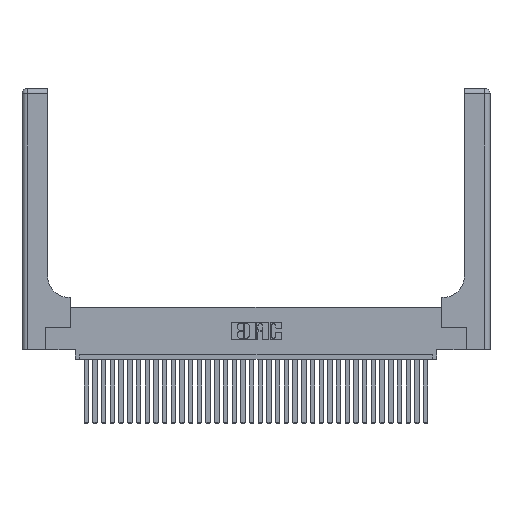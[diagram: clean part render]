
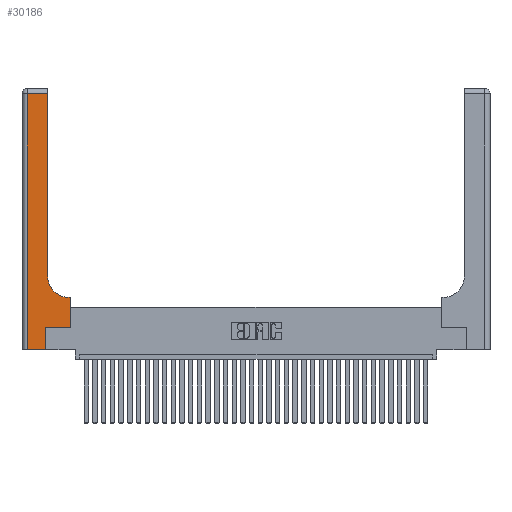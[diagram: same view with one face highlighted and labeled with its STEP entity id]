
A CAD part, top view. The second image highlights one B-rep face of the part: STEP entity #30186.
In plain terms, the highlighted planar face has unit normal (0, 0, 1).
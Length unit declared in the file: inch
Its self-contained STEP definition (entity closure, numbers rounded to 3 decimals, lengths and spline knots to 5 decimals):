
#1551 = PLANE ( 'NONE',  #24170 ) ;
#1641 = FACE_OUTER_BOUND ( 'NONE', #23028, .T. ) ;
#1851 = CIRCLE ( 'NONE', #33750, 0.25 ) ;
#2514 = ORIENTED_EDGE ( 'NONE', *, *, #33948, .T. ) ;
#2633 = EDGE_CURVE ( 'NONE', #8503, #35293, #25731, .T. ) ;
#3363 = CARTESIAN_POINT ( 'NONE',  ( 0.2915, 3., 0.37 ) ) ;
#3976 = ORIENTED_EDGE ( 'NONE', *, *, #13596, .T. ) ;
#4954 = EDGE_CURVE ( 'NONE', #15916, #24960, #19930, .T. ) ;
#4958 = EDGE_CURVE ( 'NONE', #7958, #14568, #5290, .T. ) ;
#4986 = DIRECTION ( 'NONE',  ( 0., 0., -1. ) ) ;
#5290 = LINE ( 'NONE', #32312, #18690 ) ;
#5787 = LINE ( 'NONE', #25757, #12323 ) ;
#6427 = LINE ( 'NONE', #31653, #23250 ) ;
#6730 = EDGE_CURVE ( 'NONE', #35293, #18492, #1851, .T. ) ;
#6784 = CARTESIAN_POINT ( 'NONE',  ( 0.06, 0., 0.37 ) ) ;
#6954 = CARTESIAN_POINT ( 'NONE',  ( 0.2915, 0.85, 0.37 ) ) ;
#7958 = VERTEX_POINT ( 'NONE', #24317 ) ;
#8503 = VERTEX_POINT ( 'NONE', #20651 ) ;
#8727 = DIRECTION ( 'NONE',  ( 0., 1., 0. ) ) ;
#9308 = ORIENTED_EDGE ( 'NONE', *, *, #25442, .T. ) ;
#9328 = CARTESIAN_POINT ( 'NONE',  ( 0.2915, 2.94, 0.37 ) ) ;
#9330 = ORIENTED_EDGE ( 'NONE', *, *, #6730, .T. ) ;
#9732 = CARTESIAN_POINT ( 'NONE',  ( 0.06, 2.94, 0.37 ) ) ;
#9828 = VECTOR ( 'NONE', #20749, 39.37008 ) ;
#9844 = CARTESIAN_POINT ( 'NONE',  ( 0., 3., 0.37 ) ) ;
#11902 = CARTESIAN_POINT ( 'NONE',  ( 0., 0., 0.37 ) ) ;
#12200 = ORIENTED_EDGE ( 'NONE', *, *, #29926, .T. ) ;
#12323 = VECTOR ( 'NONE', #31496, 39.37008 ) ;
#13596 = EDGE_CURVE ( 'NONE', #18492, #30036, #19755, .T. ) ;
#14226 = DIRECTION ( 'NONE',  ( -1., 0., 0. ) ) ;
#14568 = VERTEX_POINT ( 'NONE', #30795 ) ;
#15698 = CARTESIAN_POINT ( 'NONE',  ( 0.2915, 0.6, 0.37 ) ) ;
#15916 = VERTEX_POINT ( 'NONE', #9732 ) ;
#15969 = CARTESIAN_POINT ( 'NONE',  ( 0.5415, 0.6, 0.37 ) ) ;
#16258 = DIRECTION ( 'NONE',  ( 1., 0., 0. ) ) ;
#18492 = VERTEX_POINT ( 'NONE', #6954 ) ;
#18643 = CARTESIAN_POINT ( 'NONE',  ( 0.5585, 0.25, 0.37 ) ) ;
#18690 = VECTOR ( 'NONE', #21539, 39.37008 ) ;
#19100 = CARTESIAN_POINT ( 'NONE',  ( 0.5415, 0.85, 0.37 ) ) ;
#19532 = EDGE_CURVE ( 'NONE', #30036, #15916, #6427, .T. ) ;
#19755 = LINE ( 'NONE', #3363, #32232 ) ;
#19899 = VERTEX_POINT ( 'NONE', #35441 ) ;
#19930 = LINE ( 'NONE', #28637, #35369 ) ;
#20559 = LINE ( 'NONE', #11902, #32533 ) ;
#20651 = CARTESIAN_POINT ( 'NONE',  ( 0.5585, 0.6, 0.37 ) ) ;
#20749 = DIRECTION ( 'NONE',  ( -1., 0., 0. ) ) ;
#21539 = DIRECTION ( 'NONE',  ( 0., 1., 0. ) ) ;
#22475 = ORIENTED_EDGE ( 'NONE', *, *, #19532, .T. ) ;
#23028 = EDGE_LOOP ( 'NONE', ( #3976, #22475, #32896, #12200, #29825, #2514, #9308, #23126, #9330 ) ) ;
#23126 = ORIENTED_EDGE ( 'NONE', *, *, #2633, .T. ) ;
#23250 = VECTOR ( 'NONE', #23511, 39.37008 ) ;
#23511 = DIRECTION ( 'NONE',  ( -1., 0., 0. ) ) ;
#23925 = VECTOR ( 'NONE', #30034, 39.37008 ) ;
#24170 = AXIS2_PLACEMENT_3D ( 'NONE', #9844, #4986, #14226 ) ;
#24317 = CARTESIAN_POINT ( 'NONE',  ( 0.269, 0., 0.37 ) ) ;
#24960 = VERTEX_POINT ( 'NONE', #6784 ) ;
#25442 = EDGE_CURVE ( 'NONE', #19899, #8503, #33266, .T. ) ;
#25731 = LINE ( 'NONE', #15698, #9828 ) ;
#25757 = CARTESIAN_POINT ( 'NONE',  ( 0.269, 0.25, 0.37 ) ) ;
#28637 = CARTESIAN_POINT ( 'NONE',  ( 0.06, 3., 0.37 ) ) ;
#29825 = ORIENTED_EDGE ( 'NONE', *, *, #4958, .T. ) ;
#29926 = EDGE_CURVE ( 'NONE', #24960, #7958, #20559, .T. ) ;
#30034 = DIRECTION ( 'NONE',  ( 0., 1., 0. ) ) ;
#30036 = VERTEX_POINT ( 'NONE', #9328 ) ;
#30186 = ADVANCED_FACE ( 'NONE', ( #1641 ), #1551, .F. ) ;
#30795 = CARTESIAN_POINT ( 'NONE',  ( 0.269, 0.25, 0.37 ) ) ;
#31307 = DIRECTION ( 'NONE',  ( 1., 0., 0. ) ) ;
#31496 = DIRECTION ( 'NONE',  ( 1., 0., 0. ) ) ;
#31653 = CARTESIAN_POINT ( 'NONE',  ( 0., 2.94, 0.37 ) ) ;
#32232 = VECTOR ( 'NONE', #8727, 39.37008 ) ;
#32312 = CARTESIAN_POINT ( 'NONE',  ( 0.269, 0., 0.37 ) ) ;
#32533 = VECTOR ( 'NONE', #31307, 39.37008 ) ;
#32896 = ORIENTED_EDGE ( 'NONE', *, *, #4954, .T. ) ;
#33266 = LINE ( 'NONE', #18643, #23925 ) ;
#33718 = DIRECTION ( 'NONE',  ( 0., -1., 0. ) ) ;
#33750 = AXIS2_PLACEMENT_3D ( 'NONE', #19100, #35044, #16258 ) ;
#33948 = EDGE_CURVE ( 'NONE', #14568, #19899, #5787, .T. ) ;
#35044 = DIRECTION ( 'NONE',  ( 0., 0., -1. ) ) ;
#35293 = VERTEX_POINT ( 'NONE', #15969 ) ;
#35369 = VECTOR ( 'NONE', #33718, 39.37008 ) ;
#35441 = CARTESIAN_POINT ( 'NONE',  ( 0.5585, 0.25, 0.37 ) ) ;
